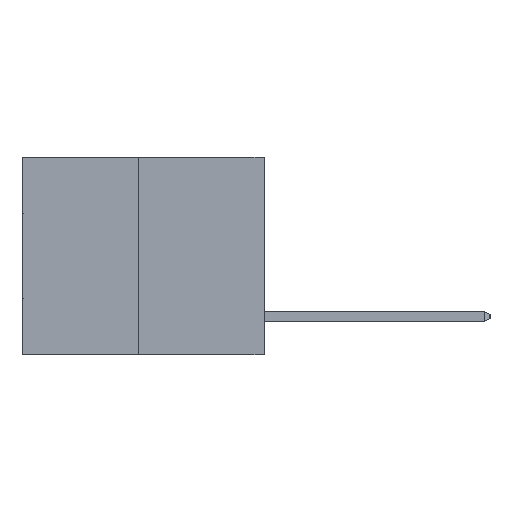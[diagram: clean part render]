
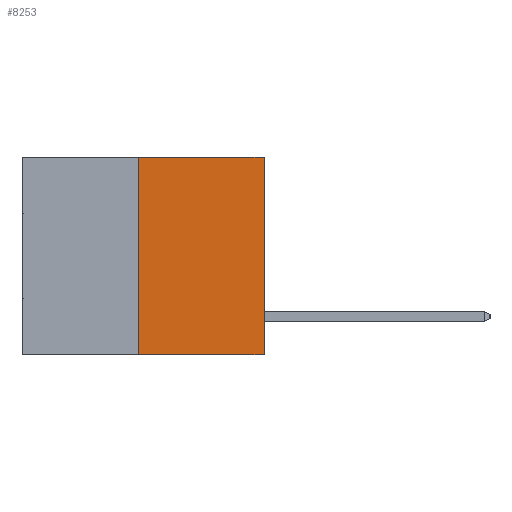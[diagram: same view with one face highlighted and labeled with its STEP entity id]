
A CAD part, left-side view. The second image highlights one B-rep face of the part: STEP entity #8253.
In plain terms, the highlighted planar face has unit normal (-1, 0, 0).
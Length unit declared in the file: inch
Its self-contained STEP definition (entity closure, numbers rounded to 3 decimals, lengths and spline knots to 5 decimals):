
#580 = VERTEX_POINT ( 'NONE', #20112 ) ;
#1141 = CARTESIAN_POINT ( 'NONE',  ( 0., 0.6, 0. ) ) ;
#1685 = CARTESIAN_POINT ( 'NONE',  ( 0., 0., 0. ) ) ;
#2570 = VERTEX_POINT ( 'NONE', #15477 ) ;
#3009 = EDGE_CURVE ( 'NONE', #2570, #15027, #21981, .T. ) ;
#4262 = CARTESIAN_POINT ( 'NONE',  ( 0., 0., 0. ) ) ;
#5069 = LINE ( 'NONE', #1141, #28357 ) ;
#5964 = EDGE_LOOP ( 'NONE', ( #26683, #30695, #26327, #28700 ) ) ;
#8253 = ADVANCED_FACE ( 'NONE', ( #16293 ), #15303, .F. ) ;
#9505 = DIRECTION ( 'NONE',  ( 0., 0., -1. ) ) ;
#10021 = CARTESIAN_POINT ( 'NONE',  ( 0., 0.6, -0.49 ) ) ;
#10708 = DIRECTION ( 'NONE',  ( 0., -1., 0. ) ) ;
#14962 = EDGE_CURVE ( 'NONE', #580, #2570, #24864, .T. ) ;
#15027 = VERTEX_POINT ( 'NONE', #4262 ) ;
#15303 = PLANE ( 'NONE',  #17894 ) ;
#15400 = LINE ( 'NONE', #21069, #17350 ) ;
#15477 = CARTESIAN_POINT ( 'NONE',  ( 0., 0., -0.49 ) ) ;
#15877 = CARTESIAN_POINT ( 'NONE',  ( 0., 0.312, 0. ) ) ;
#16293 = FACE_OUTER_BOUND ( 'NONE', #5964, .T. ) ;
#17350 = VECTOR ( 'NONE', #20966, 39.37008 ) ;
#17894 = AXIS2_PLACEMENT_3D ( 'NONE', #22662, #24152, #9505 ) ;
#19474 = EDGE_CURVE ( 'NONE', #29822, #15027, #5069, .T. ) ;
#19547 = EDGE_CURVE ( 'NONE', #580, #29822, #15400, .T. ) ;
#20112 = CARTESIAN_POINT ( 'NONE',  ( 0., 0.312, -0.49 ) ) ;
#20966 = DIRECTION ( 'NONE',  ( 0., 0., 1. ) ) ;
#21069 = CARTESIAN_POINT ( 'NONE',  ( 0., 0.312, -0.49 ) ) ;
#21981 = LINE ( 'NONE', #1685, #30371 ) ;
#22662 = CARTESIAN_POINT ( 'NONE',  ( 0., 0.6, 0. ) ) ;
#24152 = DIRECTION ( 'NONE',  ( 1., 0., 0. ) ) ;
#24864 = LINE ( 'NONE', #10021, #30579 ) ;
#26327 = ORIENTED_EDGE ( 'NONE', *, *, #3009, .T. ) ;
#26683 = ORIENTED_EDGE ( 'NONE', *, *, #19547, .F. ) ;
#27234 = DIRECTION ( 'NONE',  ( 0., -1., 0. ) ) ;
#28357 = VECTOR ( 'NONE', #10708, 39.37008 ) ;
#28700 = ORIENTED_EDGE ( 'NONE', *, *, #19474, .F. ) ;
#29822 = VERTEX_POINT ( 'NONE', #15877 ) ;
#30371 = VECTOR ( 'NONE', #30653, 39.37008 ) ;
#30579 = VECTOR ( 'NONE', #27234, 39.37008 ) ;
#30653 = DIRECTION ( 'NONE',  ( 0., 0., 1. ) ) ;
#30695 = ORIENTED_EDGE ( 'NONE', *, *, #14962, .T. ) ;
